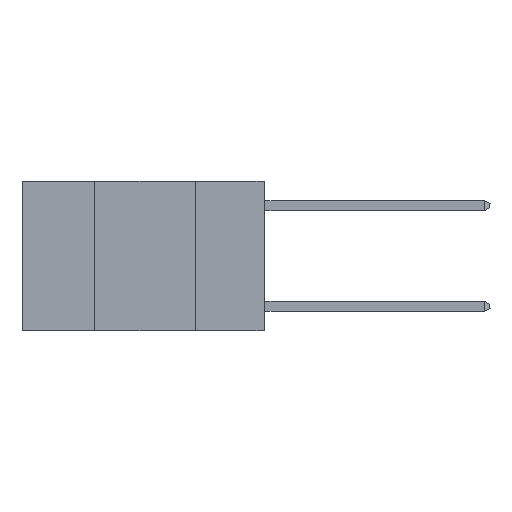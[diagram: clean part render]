
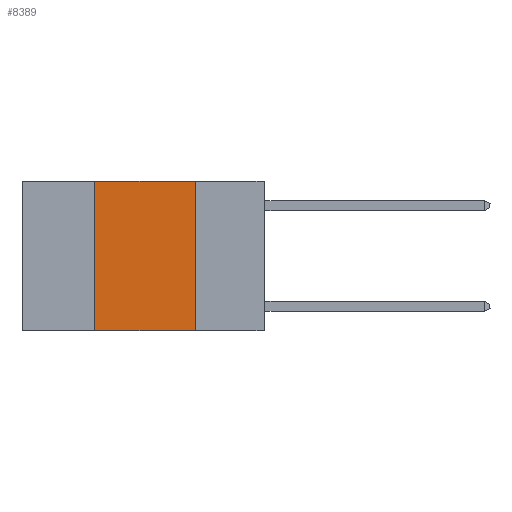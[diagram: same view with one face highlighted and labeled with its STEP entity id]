
A CAD part, left-side view. The second image highlights one B-rep face of the part: STEP entity #8389.
In plain terms, the highlighted planar face has unit normal (-1, 0, 0).
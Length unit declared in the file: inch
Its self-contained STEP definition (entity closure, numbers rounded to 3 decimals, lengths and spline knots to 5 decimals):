
#135 = VERTEX_POINT ( 'NONE', #2863 ) ;
#572 = EDGE_CURVE ( 'NONE', #4674, #1207, #3336, .T. ) ;
#599 = VECTOR ( 'NONE', #9890, 39.37008 ) ;
#807 = ORIENTED_EDGE ( 'NONE', *, *, #5246, .F. ) ;
#1074 = VECTOR ( 'NONE', #8077, 39.37008 ) ;
#1207 = VERTEX_POINT ( 'NONE', #3163 ) ;
#2051 = LINE ( 'NONE', #6451, #2768 ) ;
#2768 = VECTOR ( 'NONE', #9958, 39.37008 ) ;
#2863 = CARTESIAN_POINT ( 'NONE',  ( 0., 0.42, 0. ) ) ;
#2921 = CARTESIAN_POINT ( 'NONE',  ( 0., 0.42, -0.37 ) ) ;
#3079 = LINE ( 'NONE', #4001, #6320 ) ;
#3163 = CARTESIAN_POINT ( 'NONE',  ( 0., 0.17, -0.37 ) ) ;
#3232 = CARTESIAN_POINT ( 'NONE',  ( 0., 0.17, 0. ) ) ;
#3336 = LINE ( 'NONE', #6888, #599 ) ;
#4001 = CARTESIAN_POINT ( 'NONE',  ( 0., 0.6, 0. ) ) ;
#4242 = DIRECTION ( 'NONE',  ( 0., 0., -1. ) ) ;
#4271 = AXIS2_PLACEMENT_3D ( 'NONE', #10554, #7318, #4242 ) ;
#4365 = PLANE ( 'NONE',  #4271 ) ;
#4527 = LINE ( 'NONE', #6339, #1074 ) ;
#4674 = VERTEX_POINT ( 'NONE', #2921 ) ;
#5246 = EDGE_CURVE ( 'NONE', #11268, #1207, #4527, .T. ) ;
#5350 = EDGE_CURVE ( 'NONE', #4674, #135, #2051, .T. ) ;
#6320 = VECTOR ( 'NONE', #6624, 39.37008 ) ;
#6339 = CARTESIAN_POINT ( 'NONE',  ( 0., 0.17, 0. ) ) ;
#6451 = CARTESIAN_POINT ( 'NONE',  ( 0., 0.42, 0. ) ) ;
#6624 = DIRECTION ( 'NONE',  ( 0., -1., 0. ) ) ;
#6888 = CARTESIAN_POINT ( 'NONE',  ( 0., 0.6, -0.37 ) ) ;
#7318 = DIRECTION ( 'NONE',  ( 1., 0., 0. ) ) ;
#8077 = DIRECTION ( 'NONE',  ( 0., 0., -1. ) ) ;
#8389 = ADVANCED_FACE ( 'NONE', ( #11392 ), #4365, .F. ) ;
#8585 = ORIENTED_EDGE ( 'NONE', *, *, #8608, .F. ) ;
#8608 = EDGE_CURVE ( 'NONE', #135, #11268, #3079, .T. ) ;
#8787 = EDGE_LOOP ( 'NONE', ( #807, #8585, #9939, #9035 ) ) ;
#9035 = ORIENTED_EDGE ( 'NONE', *, *, #572, .T. ) ;
#9890 = DIRECTION ( 'NONE',  ( 0., -1., 0. ) ) ;
#9939 = ORIENTED_EDGE ( 'NONE', *, *, #5350, .F. ) ;
#9958 = DIRECTION ( 'NONE',  ( 0., 0., 1. ) ) ;
#10554 = CARTESIAN_POINT ( 'NONE',  ( 0., 0.6, 0. ) ) ;
#11268 = VERTEX_POINT ( 'NONE', #3232 ) ;
#11392 = FACE_OUTER_BOUND ( 'NONE', #8787, .T. ) ;
